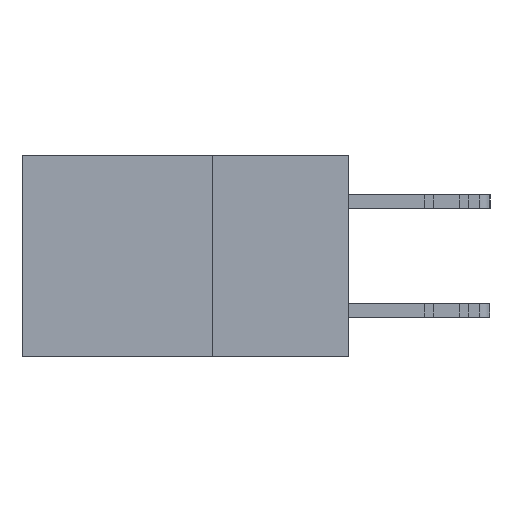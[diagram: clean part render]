
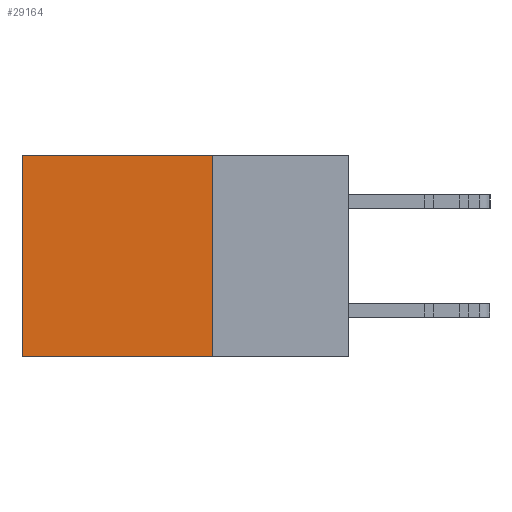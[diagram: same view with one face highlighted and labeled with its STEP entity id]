
A CAD part, left-side view. The second image highlights one B-rep face of the part: STEP entity #29164.
In plain terms, the highlighted planar face has unit normal (-1, 0, 0).
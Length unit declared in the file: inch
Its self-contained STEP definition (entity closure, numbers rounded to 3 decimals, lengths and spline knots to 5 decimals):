
#2069 = CARTESIAN_POINT ( 'NONE',  ( 0.298, 0.6, 0. ) ) ;
#2142 = VECTOR ( 'NONE', #20797, 39.37008 ) ;
#3367 = DIRECTION ( 'NONE',  ( 1., 0., 0. ) ) ;
#4374 = EDGE_CURVE ( 'NONE', #21654, #7413, #8487, .T. ) ;
#4704 = ORIENTED_EDGE ( 'NONE', *, *, #21872, .T. ) ;
#4782 = VECTOR ( 'NONE', #18904, 39.37008 ) ;
#5062 = VERTEX_POINT ( 'NONE', #25975 ) ;
#7043 = VERTEX_POINT ( 'NONE', #8467 ) ;
#7413 = VERTEX_POINT ( 'NONE', #12539 ) ;
#7874 = VECTOR ( 'NONE', #34203, 39.37008 ) ;
#8467 = CARTESIAN_POINT ( 'NONE',  ( 0.298, 0.25, -0.37 ) ) ;
#8487 = LINE ( 'NONE', #2069, #2142 ) ;
#9688 = EDGE_CURVE ( 'NONE', #7043, #7413, #11916, .T. ) ;
#11916 = LINE ( 'NONE', #16214, #4782 ) ;
#12377 = CARTESIAN_POINT ( 'NONE',  ( 0.298, 0.6, 0. ) ) ;
#12406 = CARTESIAN_POINT ( 'NONE',  ( 0.298, 0.25, 0. ) ) ;
#12539 = CARTESIAN_POINT ( 'NONE',  ( 0.298, 0.6, -0.37 ) ) ;
#13596 = ORIENTED_EDGE ( 'NONE', *, *, #4374, .T. ) ;
#14699 = EDGE_LOOP ( 'NONE', ( #13596, #20804, #20778, #4704 ) ) ;
#15790 = LINE ( 'NONE', #15815, #7874 ) ;
#15815 = CARTESIAN_POINT ( 'NONE',  ( 0.298, 0.25, 0. ) ) ;
#16214 = CARTESIAN_POINT ( 'NONE',  ( 0.298, 0.25, -0.37 ) ) ;
#17381 = EDGE_CURVE ( 'NONE', #5062, #7043, #30555, .T. ) ;
#18904 = DIRECTION ( 'NONE',  ( 0., 1., 0. ) ) ;
#19395 = PLANE ( 'NONE',  #26987 ) ;
#20778 = ORIENTED_EDGE ( 'NONE', *, *, #17381, .F. ) ;
#20797 = DIRECTION ( 'NONE',  ( 0., 0., -1. ) ) ;
#20804 = ORIENTED_EDGE ( 'NONE', *, *, #9688, .F. ) ;
#21654 = VERTEX_POINT ( 'NONE', #12377 ) ;
#21872 = EDGE_CURVE ( 'NONE', #5062, #21654, #15790, .T. ) ;
#22066 = DIRECTION ( 'NONE',  ( 0., 0., -1. ) ) ;
#23567 = VECTOR ( 'NONE', #25756, 39.37008 ) ;
#24621 = CARTESIAN_POINT ( 'NONE',  ( 0.298, 0.25, 0. ) ) ;
#25756 = DIRECTION ( 'NONE',  ( 0., 0., -1. ) ) ;
#25975 = CARTESIAN_POINT ( 'NONE',  ( 0.298, 0.25, 0. ) ) ;
#26987 = AXIS2_PLACEMENT_3D ( 'NONE', #24621, #3367, #22066 ) ;
#29164 = ADVANCED_FACE ( 'NONE', ( #33420 ), #19395, .F. ) ;
#30555 = LINE ( 'NONE', #12406, #23567 ) ;
#33420 = FACE_OUTER_BOUND ( 'NONE', #14699, .T. ) ;
#34203 = DIRECTION ( 'NONE',  ( 0., 1., 0. ) ) ;
